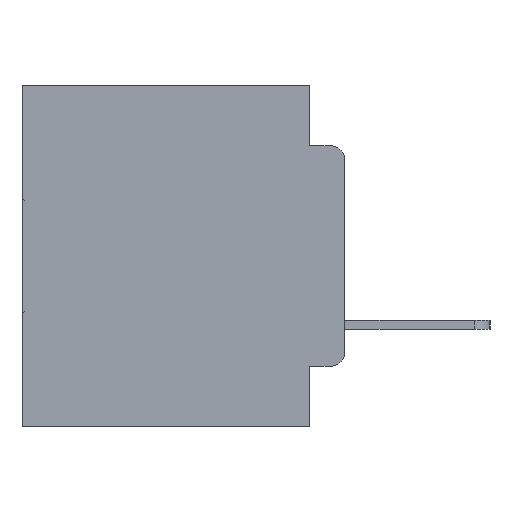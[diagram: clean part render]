
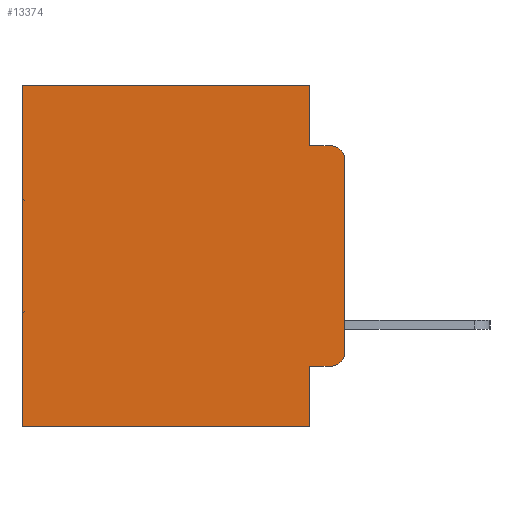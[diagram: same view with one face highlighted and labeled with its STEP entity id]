
A CAD part, left-side view. The second image highlights one B-rep face of the part: STEP entity #13374.
In plain terms, the highlighted planar face has unit normal (-1, 0, 0).
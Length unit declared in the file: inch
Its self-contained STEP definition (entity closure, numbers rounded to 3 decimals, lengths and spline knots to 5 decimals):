
#759 = CIRCLE ( 'NONE', #17334, 0.02 ) ;
#874 = LINE ( 'NONE', #3673, #7168 ) ;
#1256 = CARTESIAN_POINT ( 'NONE',  ( 0.298, 0.473, -0.5 ) ) ;
#1658 = VERTEX_POINT ( 'NONE', #4597 ) ;
#2993 = VECTOR ( 'NONE', #4752, 39.37008 ) ;
#3166 = DIRECTION ( 'NONE',  ( 0., 0., -1. ) ) ;
#3673 = CARTESIAN_POINT ( 'NONE',  ( 0.298, 0., 0. ) ) ;
#4057 = DIRECTION ( 'NONE',  ( 0., 0., -1. ) ) ;
#4159 = VERTEX_POINT ( 'NONE', #20982 ) ;
#4597 = CARTESIAN_POINT ( 'NONE',  ( 0.298, 0.051, 0. ) ) ;
#4752 = DIRECTION ( 'NONE',  ( 0., 0., -1. ) ) ;
#5026 = VERTEX_POINT ( 'NONE', #21805 ) ;
#5402 = AXIS2_PLACEMENT_3D ( 'NONE', #12692, #28995, #15173 ) ;
#5895 = VECTOR ( 'NONE', #7710, 39.37008 ) ;
#5950 = VERTEX_POINT ( 'NONE', #26764 ) ;
#5979 = CIRCLE ( 'NONE', #5402, 0.02 ) ;
#6453 = VECTOR ( 'NONE', #8472, 39.37008 ) ;
#7148 = VECTOR ( 'NONE', #27058, 39.37008 ) ;
#7168 = VECTOR ( 'NONE', #3166, 39.37008 ) ;
#7369 = EDGE_CURVE ( 'NONE', #5950, #24294, #13038, .T. ) ;
#7608 = CARTESIAN_POINT ( 'NONE',  ( 0.298, 0.051, 0. ) ) ;
#7710 = DIRECTION ( 'NONE',  ( 0., 1., 0. ) ) ;
#7747 = VERTEX_POINT ( 'NONE', #11319 ) ;
#8045 = ORIENTED_EDGE ( 'NONE', *, *, #8662, .F. ) ;
#8472 = DIRECTION ( 'NONE',  ( 0., 1., 0. ) ) ;
#8513 = CARTESIAN_POINT ( 'NONE',  ( 0.298, 0., -0.5 ) ) ;
#8662 = EDGE_CURVE ( 'NONE', #17974, #5026, #874, .T. ) ;
#9014 = EDGE_CURVE ( 'NONE', #1658, #14840, #30879, .T. ) ;
#9550 = ORIENTED_EDGE ( 'NONE', *, *, #27882, .F. ) ;
#10146 = EDGE_CURVE ( 'NONE', #7747, #5026, #759, .T. ) ;
#10544 = CARTESIAN_POINT ( 'NONE',  ( 0.298, 0.02, -0.0885 ) ) ;
#11021 = ORIENTED_EDGE ( 'NONE', *, *, #19980, .T. ) ;
#11319 = CARTESIAN_POINT ( 'NONE',  ( 0.298, 0.02, -0.4115 ) ) ;
#12588 = ORIENTED_EDGE ( 'NONE', *, *, #18660, .F. ) ;
#12692 = CARTESIAN_POINT ( 'NONE',  ( 0.298, 0.02, -0.1085 ) ) ;
#13038 = LINE ( 'NONE', #8513, #6453 ) ;
#13372 = DIRECTION ( 'NONE',  ( 1., 0., 0. ) ) ;
#13374 = ADVANCED_FACE ( 'NONE', ( #21485 ), #27442, .F. ) ;
#13665 = VECTOR ( 'NONE', #4057, 39.37008 ) ;
#14132 = CARTESIAN_POINT ( 'NONE',  ( 0.298, 0.473, 0. ) ) ;
#14177 = ORIENTED_EDGE ( 'NONE', *, *, #19740, .T. ) ;
#14203 = AXIS2_PLACEMENT_3D ( 'NONE', #23055, #13372, #29550 ) ;
#14673 = CARTESIAN_POINT ( 'NONE',  ( 0.298, 0.051, 0. ) ) ;
#14840 = VERTEX_POINT ( 'NONE', #28896 ) ;
#14862 = EDGE_CURVE ( 'NONE', #17974, #19730, #5979, .T. ) ;
#14869 = EDGE_LOOP ( 'NONE', ( #8045, #21741, #9550, #22525, #28991, #11021, #30305, #12588, #14177, #15668 ) ) ;
#15173 = DIRECTION ( 'NONE',  ( 0., 0., -1. ) ) ;
#15668 = ORIENTED_EDGE ( 'NONE', *, *, #10146, .T. ) ;
#16386 = LINE ( 'NONE', #14673, #2993 ) ;
#16744 = LINE ( 'NONE', #14132, #13665 ) ;
#16745 = CARTESIAN_POINT ( 'NONE',  ( 0.298, 0., 0. ) ) ;
#17273 = VERTEX_POINT ( 'NONE', #24707 ) ;
#17334 = AXIS2_PLACEMENT_3D ( 'NONE', #20319, #20254, #20065 ) ;
#17974 = VERTEX_POINT ( 'NONE', #26081 ) ;
#18660 = EDGE_CURVE ( 'NONE', #17273, #5950, #16386, .T. ) ;
#19730 = VERTEX_POINT ( 'NONE', #10544 ) ;
#19740 = EDGE_CURVE ( 'NONE', #17273, #7747, #24269, .T. ) ;
#19980 = EDGE_CURVE ( 'NONE', #14840, #24294, #16744, .T. ) ;
#20065 = DIRECTION ( 'NONE',  ( 0., 0., -1. ) ) ;
#20207 = LINE ( 'NONE', #24886, #7148 ) ;
#20254 = DIRECTION ( 'NONE',  ( -1., 0., 0. ) ) ;
#20319 = CARTESIAN_POINT ( 'NONE',  ( 0.298, 0.02, -0.3915 ) ) ;
#20436 = DIRECTION ( 'NONE',  ( 0., -1., 0. ) ) ;
#20982 = CARTESIAN_POINT ( 'NONE',  ( 0.298, 0.051, -0.0885 ) ) ;
#21485 = FACE_OUTER_BOUND ( 'NONE', #14869, .T. ) ;
#21741 = ORIENTED_EDGE ( 'NONE', *, *, #14862, .T. ) ;
#21805 = CARTESIAN_POINT ( 'NONE',  ( 0.298, 0., -0.3915 ) ) ;
#22041 = VECTOR ( 'NONE', #20436, 39.37008 ) ;
#22315 = DIRECTION ( 'NONE',  ( 0., 0., -1. ) ) ;
#22525 = ORIENTED_EDGE ( 'NONE', *, *, #31076, .F. ) ;
#23055 = CARTESIAN_POINT ( 'NONE',  ( 0.298, 0., 0. ) ) ;
#24269 = LINE ( 'NONE', #29265, #22041 ) ;
#24294 = VERTEX_POINT ( 'NONE', #1256 ) ;
#24707 = CARTESIAN_POINT ( 'NONE',  ( 0.298, 0.051, -0.4115 ) ) ;
#24886 = CARTESIAN_POINT ( 'NONE',  ( 0.298, 0.051, -0.0885 ) ) ;
#26081 = CARTESIAN_POINT ( 'NONE',  ( 0.298, 0., -0.1085 ) ) ;
#26764 = CARTESIAN_POINT ( 'NONE',  ( 0.298, 0.051, -0.5 ) ) ;
#27058 = DIRECTION ( 'NONE',  ( 0., -1., 0. ) ) ;
#27442 = PLANE ( 'NONE',  #14203 ) ;
#27856 = VECTOR ( 'NONE', #22315, 39.37008 ) ;
#27882 = EDGE_CURVE ( 'NONE', #4159, #19730, #20207, .T. ) ;
#28522 = LINE ( 'NONE', #7608, #27856 ) ;
#28896 = CARTESIAN_POINT ( 'NONE',  ( 0.298, 0.473, 0. ) ) ;
#28991 = ORIENTED_EDGE ( 'NONE', *, *, #9014, .T. ) ;
#28995 = DIRECTION ( 'NONE',  ( -1., 0., 0. ) ) ;
#29265 = CARTESIAN_POINT ( 'NONE',  ( 0.298, 0.051, -0.4115 ) ) ;
#29550 = DIRECTION ( 'NONE',  ( 0., 0., -1. ) ) ;
#30305 = ORIENTED_EDGE ( 'NONE', *, *, #7369, .F. ) ;
#30879 = LINE ( 'NONE', #16745, #5895 ) ;
#31076 = EDGE_CURVE ( 'NONE', #1658, #4159, #28522, .T. ) ;
